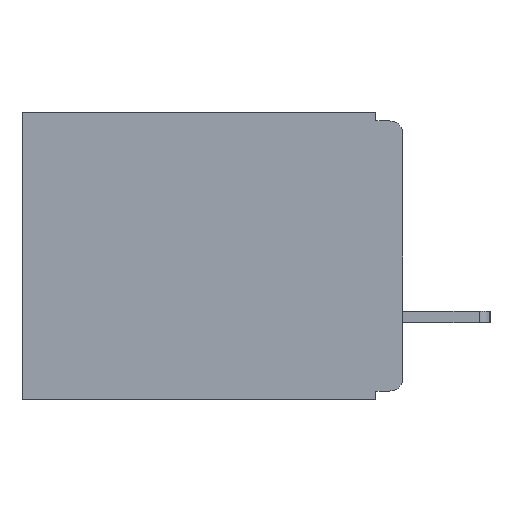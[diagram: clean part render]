
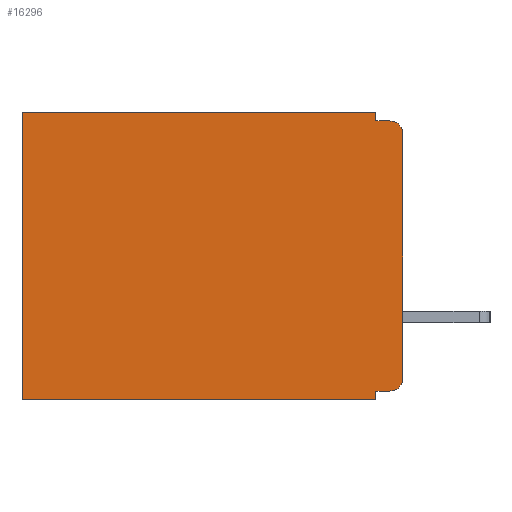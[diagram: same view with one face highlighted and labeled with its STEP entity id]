
A CAD part, left-side view. The second image highlights one B-rep face of the part: STEP entity #16296.
In plain terms, the highlighted planar face has unit normal (-1, 0, 0).
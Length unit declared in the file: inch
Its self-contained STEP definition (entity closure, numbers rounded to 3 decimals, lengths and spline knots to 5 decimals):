
#590 = EDGE_CURVE ( 'NONE', #19124, #8076, #2346, .T. ) ;
#820 = VECTOR ( 'NONE', #19351, 39.37008 ) ;
#845 = LINE ( 'NONE', #15436, #16770 ) ;
#952 = VERTEX_POINT ( 'NONE', #19810 ) ;
#965 = ORIENTED_EDGE ( 'NONE', *, *, #15846, .F. ) ;
#996 = CARTESIAN_POINT ( 'NONE',  ( 0.3, 0.031, 0. ) ) ;
#1095 = EDGE_CURVE ( 'NONE', #8076, #952, #845, .T. ) ;
#1376 = VECTOR ( 'NONE', #8222, 39.37008 ) ;
#1513 = CARTESIAN_POINT ( 'NONE',  ( 0.3, 0.031, -0.33 ) ) ;
#1596 = ORIENTED_EDGE ( 'NONE', *, *, #3376, .T. ) ;
#1616 = ORIENTED_EDGE ( 'NONE', *, *, #9580, .F. ) ;
#1681 = VERTEX_POINT ( 'NONE', #14235 ) ;
#2005 = ORIENTED_EDGE ( 'NONE', *, *, #17308, .F. ) ;
#2156 = ORIENTED_EDGE ( 'NONE', *, *, #9263, .T. ) ;
#2200 = ORIENTED_EDGE ( 'NONE', *, *, #5394, .T. ) ;
#2346 = LINE ( 'NONE', #1513, #15134 ) ;
#2351 = ORIENTED_EDGE ( 'NONE', *, *, #1095, .F. ) ;
#2399 = ORIENTED_EDGE ( 'NONE', *, *, #590, .F. ) ;
#2439 = ORIENTED_EDGE ( 'NONE', *, *, #14906, .F. ) ;
#2563 = ORIENTED_EDGE ( 'NONE', *, *, #18132, .T. ) ;
#2778 = DIRECTION ( 'NONE',  ( 0., 0., -1. ) ) ;
#3184 = AXIS2_PLACEMENT_3D ( 'NONE', #10071, #14732, #5511 ) ;
#3317 = CARTESIAN_POINT ( 'NONE',  ( 0.3, 0.015, -0.305 ) ) ;
#3338 = VECTOR ( 'NONE', #16753, 39.37008 ) ;
#3376 = EDGE_CURVE ( 'NONE', #1681, #3734, #16901, .T. ) ;
#3650 = VECTOR ( 'NONE', #10085, 39.37008 ) ;
#3734 = VERTEX_POINT ( 'NONE', #19477 ) ;
#3994 = FACE_OUTER_BOUND ( 'NONE', #14348, .T. ) ;
#4626 = DIRECTION ( 'NONE',  ( 0., 1., 0. ) ) ;
#4831 = DIRECTION ( 'NONE',  ( 0., 1., 0. ) ) ;
#4862 = DIRECTION ( 'NONE',  ( 0., 0., -1. ) ) ;
#5033 = LINE ( 'NONE', #6679, #1376 ) ;
#5394 = EDGE_CURVE ( 'NONE', #8081, #952, #19915, .T. ) ;
#5511 = DIRECTION ( 'NONE',  ( 0., 0., -1. ) ) ;
#5600 = CARTESIAN_POINT ( 'NONE',  ( 0.3, 0., -0.33 ) ) ;
#6017 = CARTESIAN_POINT ( 'NONE',  ( 0.3, 0., -0.01 ) ) ;
#6097 = AXIS2_PLACEMENT_3D ( 'NONE', #9129, #18410, #19011 ) ;
#6679 = CARTESIAN_POINT ( 'NONE',  ( 0.3, 0., 0. ) ) ;
#7019 = VERTEX_POINT ( 'NONE', #7192 ) ;
#7192 = CARTESIAN_POINT ( 'NONE',  ( 0.3, 0.015, -0.32 ) ) ;
#8076 = VERTEX_POINT ( 'NONE', #14407 ) ;
#8081 = VERTEX_POINT ( 'NONE', #9309 ) ;
#8222 = DIRECTION ( 'NONE',  ( 0., 1., 0. ) ) ;
#9129 = CARTESIAN_POINT ( 'NONE',  ( 0.3, 0.015, -0.025 ) ) ;
#9245 = CARTESIAN_POINT ( 'NONE',  ( 0.3, 0.437, -0.33 ) ) ;
#9263 = EDGE_CURVE ( 'NONE', #11273, #8081, #5033, .T. ) ;
#9309 = CARTESIAN_POINT ( 'NONE',  ( 0.3, 0.437, 0. ) ) ;
#9453 = CARTESIAN_POINT ( 'NONE',  ( 0.3, 0., -0.305 ) ) ;
#9580 = EDGE_CURVE ( 'NONE', #14040, #3734, #15113, .T. ) ;
#9663 = CIRCLE ( 'NONE', #13283, 0.015 ) ;
#10071 = CARTESIAN_POINT ( 'NONE',  ( 0.3, 0., -0.33 ) ) ;
#10085 = DIRECTION ( 'NONE',  ( 0., 0., -1. ) ) ;
#10955 = CARTESIAN_POINT ( 'NONE',  ( 0.3, 0.031, -0.01 ) ) ;
#11029 = LINE ( 'NONE', #12526, #19119 ) ;
#11273 = VERTEX_POINT ( 'NONE', #996 ) ;
#12526 = CARTESIAN_POINT ( 'NONE',  ( 0.3, 0., -0.32 ) ) ;
#13144 = PLANE ( 'NONE',  #3184 ) ;
#13283 = AXIS2_PLACEMENT_3D ( 'NONE', #3317, #14092, #4862 ) ;
#13563 = VERTEX_POINT ( 'NONE', #9453 ) ;
#13837 = LINE ( 'NONE', #16623, #17843 ) ;
#14040 = VERTEX_POINT ( 'NONE', #10955 ) ;
#14092 = DIRECTION ( 'NONE',  ( -1., 0., 0. ) ) ;
#14235 = CARTESIAN_POINT ( 'NONE',  ( 0.3, 0., -0.025 ) ) ;
#14348 = EDGE_LOOP ( 'NONE', ( #965, #1596, #1616, #2005, #2156, #2200, #2351, #2399, #2439, #2563 ) ) ;
#14407 = CARTESIAN_POINT ( 'NONE',  ( 0.3, 0.031, -0.33 ) ) ;
#14732 = DIRECTION ( 'NONE',  ( 1., 0., 0. ) ) ;
#14906 = EDGE_CURVE ( 'NONE', #7019, #19124, #11029, .T. ) ;
#15113 = LINE ( 'NONE', #6017, #3338 ) ;
#15134 = VECTOR ( 'NONE', #16727, 39.37008 ) ;
#15436 = CARTESIAN_POINT ( 'NONE',  ( 0.3, 0., -0.33 ) ) ;
#15846 = EDGE_CURVE ( 'NONE', #1681, #13563, #16745, .T. ) ;
#16296 = ADVANCED_FACE ( 'NONE', ( #3994 ), #13144, .F. ) ;
#16623 = CARTESIAN_POINT ( 'NONE',  ( 0.3, 0.031, 0. ) ) ;
#16727 = DIRECTION ( 'NONE',  ( 0., 0., -1. ) ) ;
#16745 = LINE ( 'NONE', #5600, #820 ) ;
#16753 = DIRECTION ( 'NONE',  ( 0., -1., 0. ) ) ;
#16770 = VECTOR ( 'NONE', #4626, 39.37008 ) ;
#16901 = CIRCLE ( 'NONE', #6097, 0.015 ) ;
#17308 = EDGE_CURVE ( 'NONE', #11273, #14040, #13837, .T. ) ;
#17843 = VECTOR ( 'NONE', #2778, 39.37008 ) ;
#17993 = CARTESIAN_POINT ( 'NONE',  ( 0.3, 0.031, -0.32 ) ) ;
#18132 = EDGE_CURVE ( 'NONE', #7019, #13563, #9663, .T. ) ;
#18410 = DIRECTION ( 'NONE',  ( -1., 0., 0. ) ) ;
#19011 = DIRECTION ( 'NONE',  ( 0., 0., -1. ) ) ;
#19119 = VECTOR ( 'NONE', #4831, 39.37008 ) ;
#19124 = VERTEX_POINT ( 'NONE', #17993 ) ;
#19351 = DIRECTION ( 'NONE',  ( 0., 0., -1. ) ) ;
#19477 = CARTESIAN_POINT ( 'NONE',  ( 0.3, 0.015, -0.01 ) ) ;
#19810 = CARTESIAN_POINT ( 'NONE',  ( 0.3, 0.437, -0.33 ) ) ;
#19915 = LINE ( 'NONE', #9245, #3650 ) ;
